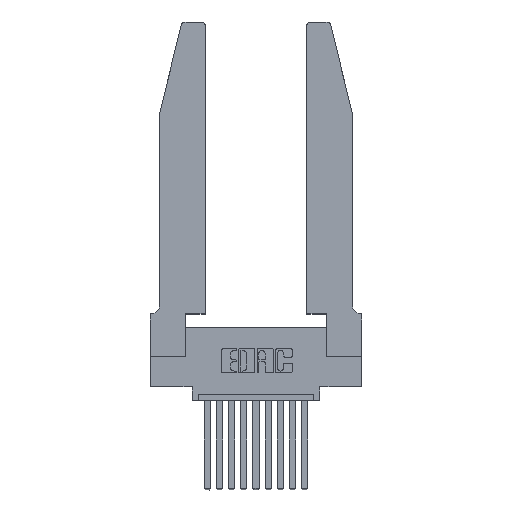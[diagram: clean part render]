
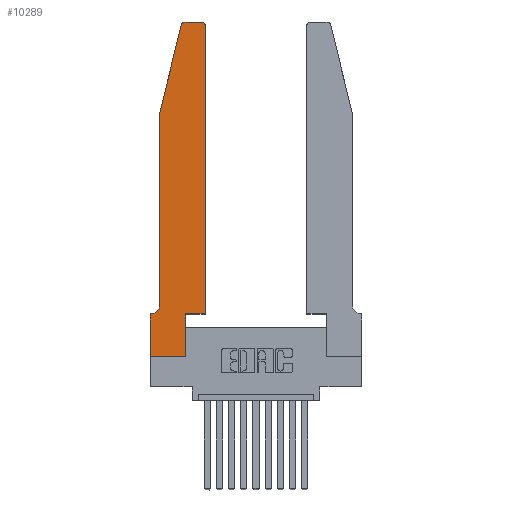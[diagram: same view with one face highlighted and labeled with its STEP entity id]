
A CAD part, top view. The second image highlights one B-rep face of the part: STEP entity #10289.
In plain terms, the highlighted planar face has unit normal (0, 0, 1).
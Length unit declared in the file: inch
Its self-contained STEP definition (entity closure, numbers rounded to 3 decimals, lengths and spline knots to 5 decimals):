
#258 = DIRECTION ( 'NONE',  ( -0.239, -0.971, 0. ) ) ;
#332 = LINE ( 'NONE', #1072, #8776 ) ;
#379 = LINE ( 'NONE', #8726, #9189 ) ;
#490 = EDGE_CURVE ( 'NONE', #6308, #10606, #379, .T. ) ;
#560 = CARTESIAN_POINT ( 'NONE',  ( 0.0055, 0.42, 0.37 ) ) ;
#592 = CARTESIAN_POINT ( 'NONE',  ( 0.25487, 2.72718, 0.37 ) ) ;
#853 = AXIS2_PLACEMENT_3D ( 'NONE', #12099, #15696, #2201 ) ;
#1027 = LINE ( 'NONE', #14980, #4499 ) ;
#1035 = DIRECTION ( 'NONE',  ( 0., -1., 0. ) ) ;
#1072 = CARTESIAN_POINT ( 'NONE',  ( 0.2865, 0.35, 0.37 ) ) ;
#1097 = LINE ( 'NONE', #2763, #13012 ) ;
#2142 = ORIENTED_EDGE ( 'NONE', *, *, #4093, .T. ) ;
#2165 = LINE ( 'NONE', #13907, #11001 ) ;
#2201 = DIRECTION ( 'NONE',  ( 1., 0., 0. ) ) ;
#2763 = CARTESIAN_POINT ( 'NONE',  ( 0.0755, 2., 0.37 ) ) ;
#2818 = ORIENTED_EDGE ( 'NONE', *, *, #7957, .T. ) ;
#2900 = EDGE_LOOP ( 'NONE', ( #8224, #10138, #9249, #2818, #8039, #9767, #13713, #4024, #2142, #14971, #7666, #13590 ) ) ;
#3070 = DIRECTION ( 'NONE',  ( -1., 0., 0. ) ) ;
#3344 = CARTESIAN_POINT ( 'NONE',  ( 0.0755, 0.42, 0.37 ) ) ;
#3697 = VECTOR ( 'NONE', #1035, 39.37008 ) ;
#3915 = VECTOR ( 'NONE', #7095, 39.37008 ) ;
#3988 = DIRECTION ( 'NONE',  ( 1., 0., 0. ) ) ;
#4024 = ORIENTED_EDGE ( 'NONE', *, *, #5695, .T. ) ;
#4070 = DIRECTION ( 'NONE',  ( 0., 1., 0. ) ) ;
#4093 = EDGE_CURVE ( 'NONE', #11505, #12239, #332, .T. ) ;
#4175 = DIRECTION ( 'NONE',  ( 0., 0., 1. ) ) ;
#4499 = VECTOR ( 'NONE', #3988, 39.37008 ) ;
#4715 = CIRCLE ( 'NONE', #10556, 0.03 ) ;
#5100 = CARTESIAN_POINT ( 'NONE',  ( 0.284, 2.72, 0.37 ) ) ;
#5335 = CARTESIAN_POINT ( 'NONE',  ( 0., 0., 0.37 ) ) ;
#5695 = EDGE_CURVE ( 'NONE', #12921, #11505, #10469, .T. ) ;
#6176 = VERTEX_POINT ( 'NONE', #8344 ) ;
#6308 = VERTEX_POINT ( 'NONE', #11404 ) ;
#6318 = CARTESIAN_POINT ( 'NONE',  ( 0.0755, 2., 0.37 ) ) ;
#6410 = DIRECTION ( 'NONE',  ( 1., 0., 0. ) ) ;
#6435 = DIRECTION ( 'NONE',  ( 0., 0., 1. ) ) ;
#6604 = EDGE_CURVE ( 'NONE', #12239, #7310, #1027, .T. ) ;
#6795 = LINE ( 'NONE', #14532, #3915 ) ;
#7014 = CIRCLE ( 'NONE', #14093, 0.03 ) ;
#7095 = DIRECTION ( 'NONE',  ( 0., -1., 0. ) ) ;
#7165 = CARTESIAN_POINT ( 'NONE',  ( 0.0755, 2., 0.37 ) ) ;
#7310 = VERTEX_POINT ( 'NONE', #10077 ) ;
#7666 = ORIENTED_EDGE ( 'NONE', *, *, #10294, .T. ) ;
#7730 = CARTESIAN_POINT ( 'NONE',  ( 0., 0.35, 0.37 ) ) ;
#7734 = DIRECTION ( 'NONE',  ( 1., 0., 0. ) ) ;
#7883 = FACE_OUTER_BOUND ( 'NONE', #2900, .T. ) ;
#7912 = LINE ( 'NONE', #7165, #3697 ) ;
#7957 = EDGE_CURVE ( 'NONE', #13892, #9590, #7912, .T. ) ;
#7965 = CARTESIAN_POINT ( 'NONE',  ( 0.2865, 0.35, 0.37 ) ) ;
#8039 = ORIENTED_EDGE ( 'NONE', *, *, #9484, .T. ) ;
#8224 = ORIENTED_EDGE ( 'NONE', *, *, #490, .T. ) ;
#8280 = VECTOR ( 'NONE', #8418, 39.37008 ) ;
#8344 = CARTESIAN_POINT ( 'NONE',  ( 0.0055, 0.35, 0.37 ) ) ;
#8418 = DIRECTION ( 'NONE',  ( 0., 1., 0. ) ) ;
#8422 = EDGE_CURVE ( 'NONE', #8771, #12921, #6795, .T. ) ;
#8726 = CARTESIAN_POINT ( 'NONE',  ( 0.2605, 2.75, 0.37 ) ) ;
#8771 = VERTEX_POINT ( 'NONE', #7730 ) ;
#8776 = VECTOR ( 'NONE', #4070, 39.37008 ) ;
#8890 = VERTEX_POINT ( 'NONE', #10347 ) ;
#8900 = VERTEX_POINT ( 'NONE', #592 ) ;
#9171 = AXIS2_PLACEMENT_3D ( 'NONE', #560, #12845, #3070 ) ;
#9189 = VECTOR ( 'NONE', #15053, 39.37008 ) ;
#9249 = ORIENTED_EDGE ( 'NONE', *, *, #13240, .T. ) ;
#9423 = EDGE_CURVE ( 'NONE', #6176, #8771, #2165, .T. ) ;
#9484 = EDGE_CURVE ( 'NONE', #9590, #6176, #11759, .T. ) ;
#9590 = VERTEX_POINT ( 'NONE', #3344 ) ;
#9767 = ORIENTED_EDGE ( 'NONE', *, *, #9423, .T. ) ;
#10077 = CARTESIAN_POINT ( 'NONE',  ( 0.4505, 0.35, 0.37 ) ) ;
#10138 = ORIENTED_EDGE ( 'NONE', *, *, #14102, .T. ) ;
#10278 = CARTESIAN_POINT ( 'NONE',  ( 0.2865, 0., 0.37 ) ) ;
#10289 = ADVANCED_FACE ( 'NONE', ( #7883 ), #13377, .T. ) ;
#10294 = EDGE_CURVE ( 'NONE', #7310, #8890, #10959, .T. ) ;
#10347 = CARTESIAN_POINT ( 'NONE',  ( 0.4505, 2.72, 0.37 ) ) ;
#10469 = LINE ( 'NONE', #5335, #11259 ) ;
#10556 = AXIS2_PLACEMENT_3D ( 'NONE', #11611, #4175, #14146 ) ;
#10606 = VERTEX_POINT ( 'NONE', #15177 ) ;
#10959 = LINE ( 'NONE', #15797, #8280 ) ;
#11001 = VECTOR ( 'NONE', #15289, 39.37008 ) ;
#11259 = VECTOR ( 'NONE', #6410, 39.37008 ) ;
#11404 = CARTESIAN_POINT ( 'NONE',  ( 0.4205, 2.75, 0.37 ) ) ;
#11505 = VERTEX_POINT ( 'NONE', #10278 ) ;
#11611 = CARTESIAN_POINT ( 'NONE',  ( 0.4205, 2.72, 0.37 ) ) ;
#11759 = CIRCLE ( 'NONE', #9171, 0.07 ) ;
#12099 = CARTESIAN_POINT ( 'NONE',  ( 0., 0.35, 0.37 ) ) ;
#12239 = VERTEX_POINT ( 'NONE', #7965 ) ;
#12845 = DIRECTION ( 'NONE',  ( 0., 0., -1. ) ) ;
#12921 = VERTEX_POINT ( 'NONE', #15898 ) ;
#13012 = VECTOR ( 'NONE', #258, 39.37008 ) ;
#13240 = EDGE_CURVE ( 'NONE', #8900, #13892, #1097, .T. ) ;
#13377 = PLANE ( 'NONE',  #853 ) ;
#13590 = ORIENTED_EDGE ( 'NONE', *, *, #13796, .T. ) ;
#13713 = ORIENTED_EDGE ( 'NONE', *, *, #8422, .T. ) ;
#13796 = EDGE_CURVE ( 'NONE', #8890, #6308, #4715, .T. ) ;
#13892 = VERTEX_POINT ( 'NONE', #6318 ) ;
#13907 = CARTESIAN_POINT ( 'NONE',  ( 0.0755, 0.35, 0.37 ) ) ;
#14093 = AXIS2_PLACEMENT_3D ( 'NONE', #5100, #6435, #7734 ) ;
#14102 = EDGE_CURVE ( 'NONE', #10606, #8900, #7014, .T. ) ;
#14146 = DIRECTION ( 'NONE',  ( 1., 0., 0. ) ) ;
#14532 = CARTESIAN_POINT ( 'NONE',  ( 0., 0., 0.37 ) ) ;
#14971 = ORIENTED_EDGE ( 'NONE', *, *, #6604, .T. ) ;
#14980 = CARTESIAN_POINT ( 'NONE',  ( 0.4505, 0.35, 0.37 ) ) ;
#15053 = DIRECTION ( 'NONE',  ( -1., 0., 0. ) ) ;
#15177 = CARTESIAN_POINT ( 'NONE',  ( 0.284, 2.75, 0.37 ) ) ;
#15289 = DIRECTION ( 'NONE',  ( -1., 0., 0. ) ) ;
#15696 = DIRECTION ( 'NONE',  ( 0., 0., 1. ) ) ;
#15797 = CARTESIAN_POINT ( 'NONE',  ( 0.4505, 0.35, 0.37 ) ) ;
#15898 = CARTESIAN_POINT ( 'NONE',  ( 0., 0., 0.37 ) ) ;
